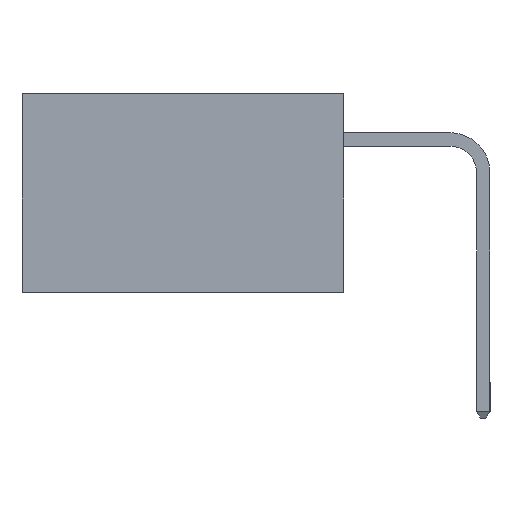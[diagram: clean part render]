
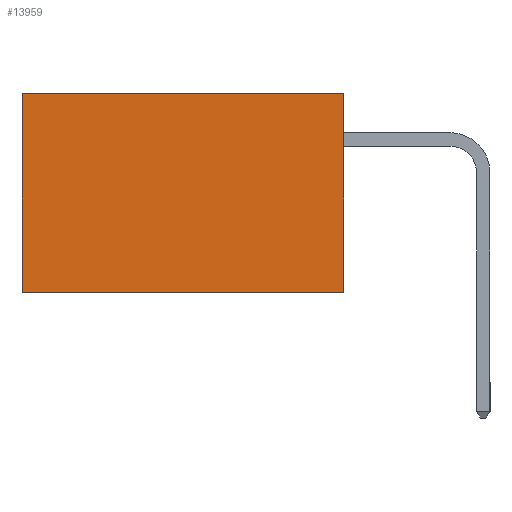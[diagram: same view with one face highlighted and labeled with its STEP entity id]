
A CAD part, left-side view. The second image highlights one B-rep face of the part: STEP entity #13959.
In plain terms, the highlighted planar face has unit normal (-1, 0, 0).
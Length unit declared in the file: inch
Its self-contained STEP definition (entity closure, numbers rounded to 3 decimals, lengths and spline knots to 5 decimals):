
#314 = CARTESIAN_POINT ( 'NONE',  ( 0.298, 0., 0. ) ) ;
#427 = EDGE_CURVE ( 'NONE', #3771, #1511, #14378, .T. ) ;
#498 = CARTESIAN_POINT ( 'NONE',  ( 0.298, 0.6, 0. ) ) ;
#502 = CARTESIAN_POINT ( 'NONE',  ( 0.298, 0., 0. ) ) ;
#991 = EDGE_CURVE ( 'NONE', #15444, #1511, #10589, .T. ) ;
#1511 = VERTEX_POINT ( 'NONE', #5368 ) ;
#2462 = DIRECTION ( 'NONE',  ( 0., 0., -1. ) ) ;
#3160 = DIRECTION ( 'NONE',  ( 1., 0., 0. ) ) ;
#3612 = LINE ( 'NONE', #7793, #13226 ) ;
#3771 = VERTEX_POINT ( 'NONE', #9625 ) ;
#3808 = EDGE_CURVE ( 'NONE', #10867, #15444, #7530, .T. ) ;
#4388 = VECTOR ( 'NONE', #8909, 39.37008 ) ;
#5368 = CARTESIAN_POINT ( 'NONE',  ( 0.298, 0.6, -0.37 ) ) ;
#6882 = VECTOR ( 'NONE', #2462, 39.37008 ) ;
#7530 = LINE ( 'NONE', #10045, #13800 ) ;
#7793 = CARTESIAN_POINT ( 'NONE',  ( 0.298, 0., 0. ) ) ;
#8081 = EDGE_LOOP ( 'NONE', ( #12712, #14918, #11246, #13343 ) ) ;
#8660 = DIRECTION ( 'NONE',  ( 0., 1., 0. ) ) ;
#8842 = EDGE_CURVE ( 'NONE', #10867, #3771, #3612, .T. ) ;
#8909 = DIRECTION ( 'NONE',  ( 0., 1., 0. ) ) ;
#9198 = AXIS2_PLACEMENT_3D ( 'NONE', #502, #3160, #11932 ) ;
#9625 = CARTESIAN_POINT ( 'NONE',  ( 0.298, 0., -0.37 ) ) ;
#9646 = DIRECTION ( 'NONE',  ( 0., 0., -1. ) ) ;
#10045 = CARTESIAN_POINT ( 'NONE',  ( 0.298, 0., 0. ) ) ;
#10356 = FACE_OUTER_BOUND ( 'NONE', #8081, .T. ) ;
#10589 = LINE ( 'NONE', #13632, #6882 ) ;
#10680 = PLANE ( 'NONE',  #9198 ) ;
#10867 = VERTEX_POINT ( 'NONE', #314 ) ;
#11246 = ORIENTED_EDGE ( 'NONE', *, *, #8842, .F. ) ;
#11932 = DIRECTION ( 'NONE',  ( 0., 0., -1. ) ) ;
#12317 = CARTESIAN_POINT ( 'NONE',  ( 0.298, 0., -0.37 ) ) ;
#12712 = ORIENTED_EDGE ( 'NONE', *, *, #991, .T. ) ;
#13226 = VECTOR ( 'NONE', #9646, 39.37008 ) ;
#13343 = ORIENTED_EDGE ( 'NONE', *, *, #3808, .T. ) ;
#13632 = CARTESIAN_POINT ( 'NONE',  ( 0.298, 0.6, 0. ) ) ;
#13800 = VECTOR ( 'NONE', #8660, 39.37008 ) ;
#13959 = ADVANCED_FACE ( 'NONE', ( #10356 ), #10680, .F. ) ;
#14378 = LINE ( 'NONE', #12317, #4388 ) ;
#14918 = ORIENTED_EDGE ( 'NONE', *, *, #427, .F. ) ;
#15444 = VERTEX_POINT ( 'NONE', #498 ) ;
